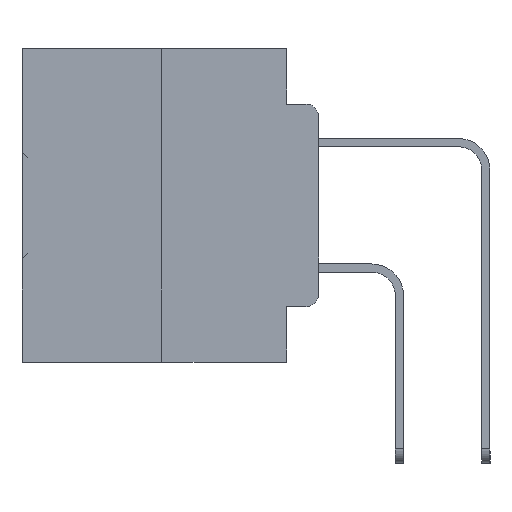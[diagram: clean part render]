
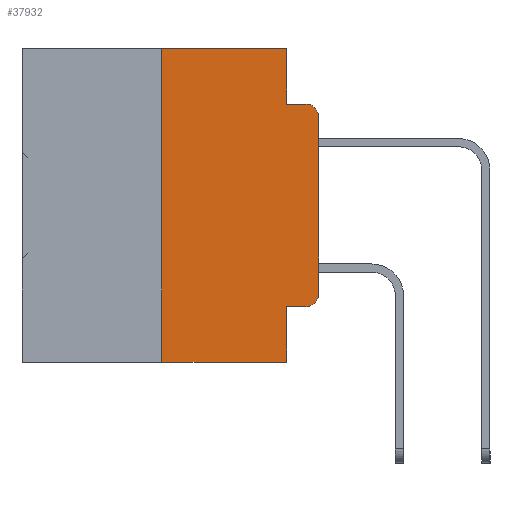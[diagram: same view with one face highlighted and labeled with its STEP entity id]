
A CAD part, left-side view. The second image highlights one B-rep face of the part: STEP entity #37932.
In plain terms, the highlighted planar face has unit normal (-1, 0, 0).
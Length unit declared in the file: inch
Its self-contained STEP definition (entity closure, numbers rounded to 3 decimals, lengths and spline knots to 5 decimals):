
#96 = DIRECTION ( 'NONE',  ( -1., 0., 0. ) ) ;
#107 = VERTEX_POINT ( 'NONE', #19494 ) ;
#1579 = VERTEX_POINT ( 'NONE', #21747 ) ;
#2417 = DIRECTION ( 'NONE',  ( 0., 0., 1. ) ) ;
#2709 = ORIENTED_EDGE ( 'NONE', *, *, #9508, .T. ) ;
#2850 = VERTEX_POINT ( 'NONE', #14339 ) ;
#4258 = VERTEX_POINT ( 'NONE', #8820 ) ;
#4892 = LINE ( 'NONE', #29430, #6789 ) ;
#4945 = LINE ( 'NONE', #35734, #33426 ) ;
#5491 = EDGE_CURVE ( 'NONE', #2850, #30387, #12052, .T. ) ;
#6789 = VECTOR ( 'NONE', #15091, 39.37008 ) ;
#6958 = ORIENTED_EDGE ( 'NONE', *, *, #5491, .F. ) ;
#7240 = CARTESIAN_POINT ( 'NONE',  ( 0., 0., 0. ) ) ;
#7318 = CARTESIAN_POINT ( 'NONE',  ( 0., 0.02, -0.3915 ) ) ;
#7527 = EDGE_CURVE ( 'NONE', #107, #30387, #30293, .T. ) ;
#8710 = PLANE ( 'NONE',  #19554 ) ;
#8820 = CARTESIAN_POINT ( 'NONE',  ( 0., 0.051, -0.4115 ) ) ;
#9508 = EDGE_CURVE ( 'NONE', #24604, #107, #16889, .T. ) ;
#9882 = DIRECTION ( 'NONE',  ( 0., 0., -1. ) ) ;
#10301 = DIRECTION ( 'NONE',  ( 0., 0., -1. ) ) ;
#11659 = DIRECTION ( 'NONE',  ( 1., 0., 0. ) ) ;
#11727 = VECTOR ( 'NONE', #30860, 39.37008 ) ;
#11862 = VECTOR ( 'NONE', #2417, 39.37008 ) ;
#12027 = VERTEX_POINT ( 'NONE', #18584 ) ;
#12052 = LINE ( 'NONE', #35309, #27707 ) ;
#12679 = VERTEX_POINT ( 'NONE', #12710 ) ;
#12710 = CARTESIAN_POINT ( 'NONE',  ( 0., 0.02, -0.4115 ) ) ;
#12735 = CARTESIAN_POINT ( 'NONE',  ( 0., 0.051, 0. ) ) ;
#12930 = CARTESIAN_POINT ( 'NONE',  ( 0., 0.051, -0.5 ) ) ;
#14339 = CARTESIAN_POINT ( 'NONE',  ( 0., 0.051, -0.0885 ) ) ;
#15091 = DIRECTION ( 'NONE',  ( 0., -1., 0. ) ) ;
#16889 = LINE ( 'NONE', #7240, #32394 ) ;
#17353 = DIRECTION ( 'NONE',  ( 0., 0., -1. ) ) ;
#17942 = CARTESIAN_POINT ( 'NONE',  ( 0., 0.02, -0.1085 ) ) ;
#18086 = ORIENTED_EDGE ( 'NONE', *, *, #35699, .F. ) ;
#18584 = CARTESIAN_POINT ( 'NONE',  ( 0., 0.25, 0. ) ) ;
#19180 = CARTESIAN_POINT ( 'NONE',  ( 0., 0.051, -0.4115 ) ) ;
#19494 = CARTESIAN_POINT ( 'NONE',  ( 0., 0., -0.1085 ) ) ;
#19554 = AXIS2_PLACEMENT_3D ( 'NONE', #20474, #11659, #32127 ) ;
#19599 = VERTEX_POINT ( 'NONE', #12930 ) ;
#19628 = LINE ( 'NONE', #19180, #11727 ) ;
#20176 = EDGE_CURVE ( 'NONE', #12679, #24604, #32923, .T. ) ;
#20236 = CARTESIAN_POINT ( 'NONE',  ( 0., 0.25, 0. ) ) ;
#20474 = CARTESIAN_POINT ( 'NONE',  ( 0., 0.473, 0. ) ) ;
#20904 = DIRECTION ( 'NONE',  ( 0., 0., -1. ) ) ;
#21319 = DIRECTION ( 'NONE',  ( 0., -1., 0. ) ) ;
#21747 = CARTESIAN_POINT ( 'NONE',  ( 0., 0.051, 0. ) ) ;
#21901 = EDGE_LOOP ( 'NONE', ( #2709, #28144, #6958, #18086, #23601, #24544, #26367, #37616, #27708, #37152 ) ) ;
#22148 = EDGE_CURVE ( 'NONE', #4258, #12679, #19628, .T. ) ;
#22863 = CARTESIAN_POINT ( 'NONE',  ( 0., 0., -0.3915 ) ) ;
#23601 = ORIENTED_EDGE ( 'NONE', *, *, #32860, .F. ) ;
#24544 = ORIENTED_EDGE ( 'NONE', *, *, #33786, .F. ) ;
#24604 = VERTEX_POINT ( 'NONE', #22863 ) ;
#24777 = AXIS2_PLACEMENT_3D ( 'NONE', #7318, #27925, #10301 ) ;
#24814 = EDGE_CURVE ( 'NONE', #25686, #19599, #4892, .T. ) ;
#25084 = CARTESIAN_POINT ( 'NONE',  ( 0., 0.25, -0.5 ) ) ;
#25415 = LINE ( 'NONE', #34785, #31257 ) ;
#25686 = VERTEX_POINT ( 'NONE', #25084 ) ;
#26367 = ORIENTED_EDGE ( 'NONE', *, *, #24814, .T. ) ;
#26611 = LINE ( 'NONE', #20236, #11862 ) ;
#26629 = DIRECTION ( 'NONE',  ( 0., -1., 0. ) ) ;
#27707 = VECTOR ( 'NONE', #26629, 39.37008 ) ;
#27708 = ORIENTED_EDGE ( 'NONE', *, *, #22148, .T. ) ;
#27925 = DIRECTION ( 'NONE',  ( -1., 0., 0. ) ) ;
#28144 = ORIENTED_EDGE ( 'NONE', *, *, #7527, .T. ) ;
#28571 = AXIS2_PLACEMENT_3D ( 'NONE', #17942, #96, #20904 ) ;
#29430 = CARTESIAN_POINT ( 'NONE',  ( 0., 0.473, -0.5 ) ) ;
#30293 = CIRCLE ( 'NONE', #28571, 0.02 ) ;
#30387 = VERTEX_POINT ( 'NONE', #30704 ) ;
#30449 = LINE ( 'NONE', #12735, #36310 ) ;
#30704 = CARTESIAN_POINT ( 'NONE',  ( 0., 0.02, -0.0885 ) ) ;
#30860 = DIRECTION ( 'NONE',  ( 0., -1., 0. ) ) ;
#31257 = VECTOR ( 'NONE', #17353, 39.37008 ) ;
#31828 = EDGE_CURVE ( 'NONE', #4258, #19599, #25415, .T. ) ;
#32127 = DIRECTION ( 'NONE',  ( 0., 0., -1. ) ) ;
#32394 = VECTOR ( 'NONE', #36526, 39.37008 ) ;
#32860 = EDGE_CURVE ( 'NONE', #12027, #1579, #4945, .T. ) ;
#32923 = CIRCLE ( 'NONE', #24777, 0.02 ) ;
#33426 = VECTOR ( 'NONE', #21319, 39.37008 ) ;
#33786 = EDGE_CURVE ( 'NONE', #25686, #12027, #26611, .T. ) ;
#34334 = FACE_OUTER_BOUND ( 'NONE', #21901, .T. ) ;
#34785 = CARTESIAN_POINT ( 'NONE',  ( 0., 0.051, 0. ) ) ;
#35309 = CARTESIAN_POINT ( 'NONE',  ( 0., 0.051, -0.0885 ) ) ;
#35699 = EDGE_CURVE ( 'NONE', #1579, #2850, #30449, .T. ) ;
#35734 = CARTESIAN_POINT ( 'NONE',  ( 0., 0.473, 0. ) ) ;
#36310 = VECTOR ( 'NONE', #9882, 39.37008 ) ;
#36526 = DIRECTION ( 'NONE',  ( 0., 0., 1. ) ) ;
#37152 = ORIENTED_EDGE ( 'NONE', *, *, #20176, .T. ) ;
#37616 = ORIENTED_EDGE ( 'NONE', *, *, #31828, .F. ) ;
#37932 = ADVANCED_FACE ( 'NONE', ( #34334 ), #8710, .F. ) ;
